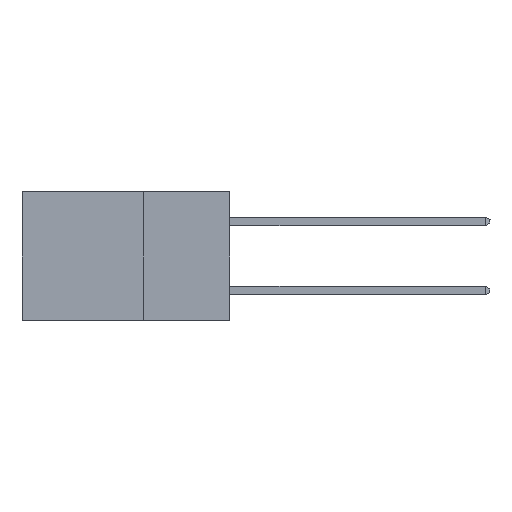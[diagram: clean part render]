
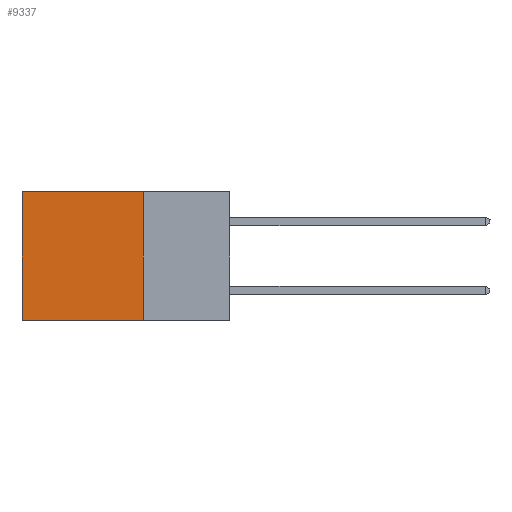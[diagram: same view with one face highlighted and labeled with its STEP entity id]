
A CAD part, left-side view. The second image highlights one B-rep face of the part: STEP entity #9337.
In plain terms, the highlighted planar face has unit normal (-1, 0, 0).
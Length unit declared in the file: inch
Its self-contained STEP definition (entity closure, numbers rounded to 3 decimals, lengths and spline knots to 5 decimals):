
#286 = DIRECTION ( 'NONE',  ( 0., 0., -1. ) ) ;
#1078 = AXIS2_PLACEMENT_3D ( 'NONE', #1562, #7055, #286 ) ;
#1289 = PLANE ( 'NONE',  #1078 ) ;
#1372 = EDGE_CURVE ( 'NONE', #3708, #7213, #11779, .T. ) ;
#1414 = EDGE_LOOP ( 'NONE', ( #8597, #6149, #8747, #15327 ) ) ;
#1562 = CARTESIAN_POINT ( 'NONE',  ( 0.2615, 0.25, -0.37 ) ) ;
#1879 = CARTESIAN_POINT ( 'NONE',  ( 0.2615, 0.25, -0.37 ) ) ;
#2147 = DIRECTION ( 'NONE',  ( 0., 0., -1. ) ) ;
#3708 = VERTEX_POINT ( 'NONE', #6968 ) ;
#3920 = VECTOR ( 'NONE', #4293, 39.37008 ) ;
#4293 = DIRECTION ( 'NONE',  ( 0., 1., 0. ) ) ;
#4905 = DIRECTION ( 'NONE',  ( 0., 1., 0. ) ) ;
#5703 = FACE_OUTER_BOUND ( 'NONE', #1414, .T. ) ;
#6090 = CARTESIAN_POINT ( 'NONE',  ( 0.2615, 0.25, -0.37 ) ) ;
#6149 = ORIENTED_EDGE ( 'NONE', *, *, #6446, .F. ) ;
#6446 = EDGE_CURVE ( 'NONE', #7213, #7467, #13896, .T. ) ;
#6968 = CARTESIAN_POINT ( 'NONE',  ( 0.2615, 0.25, 0. ) ) ;
#7055 = DIRECTION ( 'NONE',  ( 1., 0., 0. ) ) ;
#7141 = VECTOR ( 'NONE', #2147, 39.37008 ) ;
#7213 = VERTEX_POINT ( 'NONE', #6090 ) ;
#7246 = CARTESIAN_POINT ( 'NONE',  ( 0.2615, 0.25, -0.37 ) ) ;
#7467 = VERTEX_POINT ( 'NONE', #12190 ) ;
#7645 = LINE ( 'NONE', #12863, #7141 ) ;
#7680 = CARTESIAN_POINT ( 'NONE',  ( 0.2615, 0.25, 0. ) ) ;
#8193 = EDGE_CURVE ( 'NONE', #10361, #7467, #7645, .T. ) ;
#8597 = ORIENTED_EDGE ( 'NONE', *, *, #8193, .T. ) ;
#8747 = ORIENTED_EDGE ( 'NONE', *, *, #1372, .F. ) ;
#9337 = ADVANCED_FACE ( 'NONE', ( #5703 ), #1289, .F. ) ;
#10361 = VERTEX_POINT ( 'NONE', #16960 ) ;
#10429 = DIRECTION ( 'NONE',  ( 0., 0., -1. ) ) ;
#11779 = LINE ( 'NONE', #1879, #17564 ) ;
#11971 = EDGE_CURVE ( 'NONE', #3708, #10361, #17223, .T. ) ;
#12190 = CARTESIAN_POINT ( 'NONE',  ( 0.2615, 0.6, -0.37 ) ) ;
#12863 = CARTESIAN_POINT ( 'NONE',  ( 0.2615, 0.6, -0.37 ) ) ;
#13896 = LINE ( 'NONE', #7246, #3920 ) ;
#15327 = ORIENTED_EDGE ( 'NONE', *, *, #11971, .T. ) ;
#15783 = VECTOR ( 'NONE', #4905, 39.37008 ) ;
#16960 = CARTESIAN_POINT ( 'NONE',  ( 0.2615, 0.6, 0. ) ) ;
#17223 = LINE ( 'NONE', #7680, #15783 ) ;
#17564 = VECTOR ( 'NONE', #10429, 39.37008 ) ;
